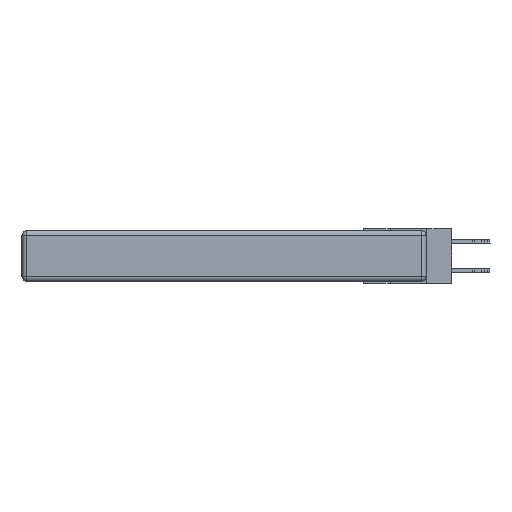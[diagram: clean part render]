
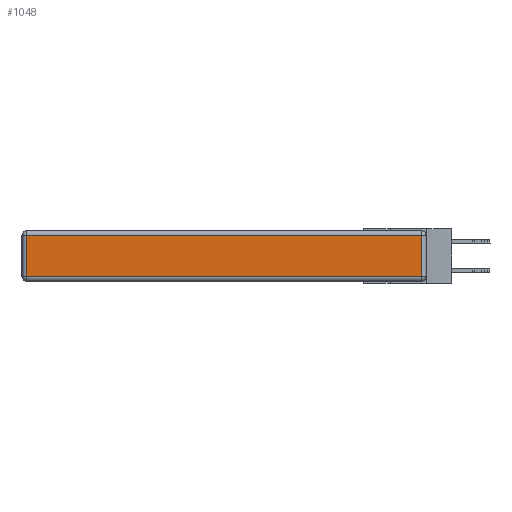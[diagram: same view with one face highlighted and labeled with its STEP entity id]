
A CAD part, left-side view. The second image highlights one B-rep face of the part: STEP entity #1048.
In plain terms, the highlighted planar face has unit normal (-1, 0, 0).
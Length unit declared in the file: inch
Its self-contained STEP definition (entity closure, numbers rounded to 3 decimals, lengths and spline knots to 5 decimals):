
#1048 = ADVANCED_FACE ( 'NONE', ( #30327 ), #13773, .T. ) ;
#1151 = DIRECTION ( 'NONE',  ( -1., 0., 0. ) ) ;
#4110 = DIRECTION ( 'NONE',  ( 0., -1., 0. ) ) ;
#4456 = DIRECTION ( 'NONE',  ( 0., 0., -1. ) ) ;
#4837 = EDGE_LOOP ( 'NONE', ( #31505, #31333, #15571, #5279 ) ) ;
#5180 = LINE ( 'NONE', #6559, #30540 ) ;
#5279 = ORIENTED_EDGE ( 'NONE', *, *, #17642, .T. ) ;
#5798 = EDGE_CURVE ( 'NONE', #20179, #24316, #29885, .T. ) ;
#6559 = CARTESIAN_POINT ( 'NONE',  ( 0., 0., -0.313 ) ) ;
#10148 = CARTESIAN_POINT ( 'NONE',  ( 0., 0.03, -0.313 ) ) ;
#11580 = CARTESIAN_POINT ( 'NONE',  ( 0., 0.03, -0.343 ) ) ;
#11891 = EDGE_CURVE ( 'NONE', #26625, #15549, #5180, .T. ) ;
#13773 = PLANE ( 'NONE',  #20823 ) ;
#15549 = VERTEX_POINT ( 'NONE', #10148 ) ;
#15571 = ORIENTED_EDGE ( 'NONE', *, *, #5798, .T. ) ;
#17445 = VECTOR ( 'NONE', #4456, 39.37008 ) ;
#17567 = CARTESIAN_POINT ( 'NONE',  ( 0., 2.72, -0.03 ) ) ;
#17642 = EDGE_CURVE ( 'NONE', #24316, #26625, #24964, .T. ) ;
#18264 = LINE ( 'NONE', #11580, #28183 ) ;
#19223 = CARTESIAN_POINT ( 'NONE',  ( 0., 0., -0.343 ) ) ;
#20179 = VERTEX_POINT ( 'NONE', #27966 ) ;
#20823 = AXIS2_PLACEMENT_3D ( 'NONE', #19223, #1151, #26527 ) ;
#21020 = EDGE_CURVE ( 'NONE', #15549, #20179, #18264, .T. ) ;
#24118 = DIRECTION ( 'NONE',  ( 0., 1., 0. ) ) ;
#24316 = VERTEX_POINT ( 'NONE', #17567 ) ;
#24964 = LINE ( 'NONE', #27302, #17445 ) ;
#26527 = DIRECTION ( 'NONE',  ( 0., 0., 1. ) ) ;
#26625 = VERTEX_POINT ( 'NONE', #27678 ) ;
#26887 = CARTESIAN_POINT ( 'NONE',  ( 0., 2.75, -0.03 ) ) ;
#27302 = CARTESIAN_POINT ( 'NONE',  ( 0., 2.72, -0.343 ) ) ;
#27542 = VECTOR ( 'NONE', #24118, 39.37008 ) ;
#27678 = CARTESIAN_POINT ( 'NONE',  ( 0., 2.72, -0.313 ) ) ;
#27966 = CARTESIAN_POINT ( 'NONE',  ( 0., 0.03, -0.03 ) ) ;
#28183 = VECTOR ( 'NONE', #29643, 39.37008 ) ;
#29643 = DIRECTION ( 'NONE',  ( 0., 0., 1. ) ) ;
#29885 = LINE ( 'NONE', #26887, #27542 ) ;
#30327 = FACE_OUTER_BOUND ( 'NONE', #4837, .T. ) ;
#30540 = VECTOR ( 'NONE', #4110, 39.37008 ) ;
#31333 = ORIENTED_EDGE ( 'NONE', *, *, #21020, .T. ) ;
#31505 = ORIENTED_EDGE ( 'NONE', *, *, #11891, .T. ) ;
